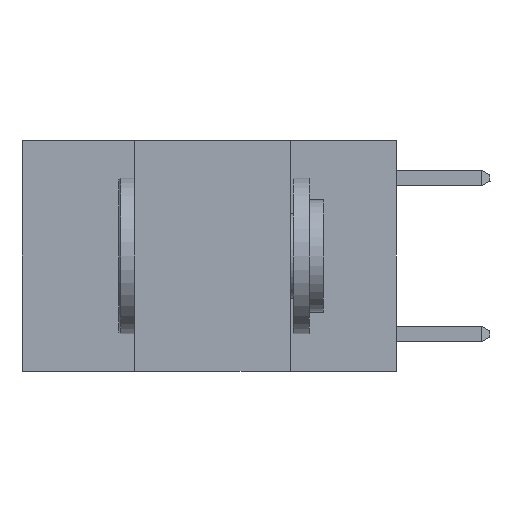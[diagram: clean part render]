
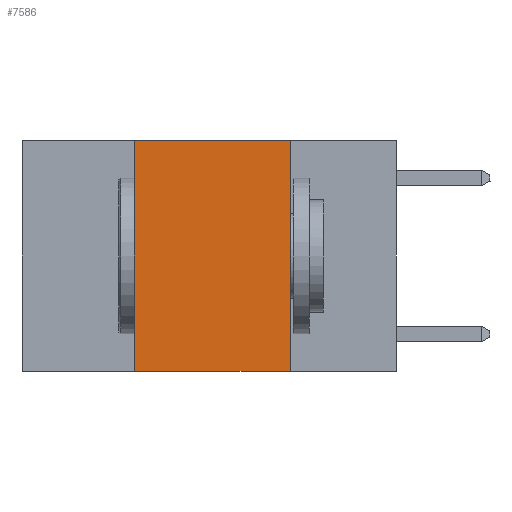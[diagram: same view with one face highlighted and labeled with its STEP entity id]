
A CAD part, left-side view. The second image highlights one B-rep face of the part: STEP entity #7586.
In plain terms, the highlighted planar face has unit normal (-1, 0, 0).
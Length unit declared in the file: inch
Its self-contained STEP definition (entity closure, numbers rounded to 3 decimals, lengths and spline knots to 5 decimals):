
#676 = CARTESIAN_POINT ( 'NONE',  ( 0., 0.42, 0. ) ) ;
#769 = VECTOR ( 'NONE', #5158, 39.37008 ) ;
#783 = LINE ( 'NONE', #6950, #769 ) ;
#1462 = VERTEX_POINT ( 'NONE', #1808 ) ;
#1808 = CARTESIAN_POINT ( 'NONE',  ( 0., 0.17, -0.37 ) ) ;
#2895 = DIRECTION ( 'NONE',  ( 0., 0., -1. ) ) ;
#2937 = AXIS2_PLACEMENT_3D ( 'NONE', #3123, #2983, #2895 ) ;
#2940 = VERTEX_POINT ( 'NONE', #676 ) ;
#2983 = DIRECTION ( 'NONE',  ( 1., 0., 0. ) ) ;
#3051 = ORIENTED_EDGE ( 'NONE', *, *, #3912, .T. ) ;
#3123 = CARTESIAN_POINT ( 'NONE',  ( 0., 0.6, 0. ) ) ;
#3197 = VERTEX_POINT ( 'NONE', #8842 ) ;
#3368 = PLANE ( 'NONE',  #2937 ) ;
#3480 = LINE ( 'NONE', #6655, #3496 ) ;
#3496 = VECTOR ( 'NONE', #6627, 39.37008 ) ;
#3543 = EDGE_CURVE ( 'NONE', #2940, #9572, #783, .T. ) ;
#3666 = CARTESIAN_POINT ( 'NONE',  ( 0., 0.17, 0. ) ) ;
#3912 = EDGE_CURVE ( 'NONE', #3197, #1462, #8806, .T. ) ;
#4042 = DIRECTION ( 'NONE',  ( 0., -1., 0. ) ) ;
#4558 = EDGE_LOOP ( 'NONE', ( #7047, #5249, #9283, #3051 ) ) ;
#5158 = DIRECTION ( 'NONE',  ( 0., -1., 0. ) ) ;
#5209 = CARTESIAN_POINT ( 'NONE',  ( 0., 0.42, 0. ) ) ;
#5249 = ORIENTED_EDGE ( 'NONE', *, *, #3543, .F. ) ;
#5951 = DIRECTION ( 'NONE',  ( 0., 0., 1. ) ) ;
#6103 = FACE_OUTER_BOUND ( 'NONE', #4558, .T. ) ;
#6627 = DIRECTION ( 'NONE',  ( 0., 0., -1. ) ) ;
#6655 = CARTESIAN_POINT ( 'NONE',  ( 0., 0.17, 0. ) ) ;
#6800 = EDGE_CURVE ( 'NONE', #3197, #2940, #8378, .T. ) ;
#6950 = CARTESIAN_POINT ( 'NONE',  ( 0., 0.6, 0. ) ) ;
#7047 = ORIENTED_EDGE ( 'NONE', *, *, #8244, .F. ) ;
#7467 = CARTESIAN_POINT ( 'NONE',  ( 0., 0.6, -0.37 ) ) ;
#7586 = ADVANCED_FACE ( 'NONE', ( #6103 ), #3368, .F. ) ;
#8244 = EDGE_CURVE ( 'NONE', #9572, #1462, #3480, .T. ) ;
#8371 = VECTOR ( 'NONE', #5951, 39.37008 ) ;
#8378 = LINE ( 'NONE', #5209, #8371 ) ;
#8806 = LINE ( 'NONE', #7467, #8820 ) ;
#8820 = VECTOR ( 'NONE', #4042, 39.37008 ) ;
#8842 = CARTESIAN_POINT ( 'NONE',  ( 0., 0.42, -0.37 ) ) ;
#9283 = ORIENTED_EDGE ( 'NONE', *, *, #6800, .F. ) ;
#9572 = VERTEX_POINT ( 'NONE', #3666 ) ;
